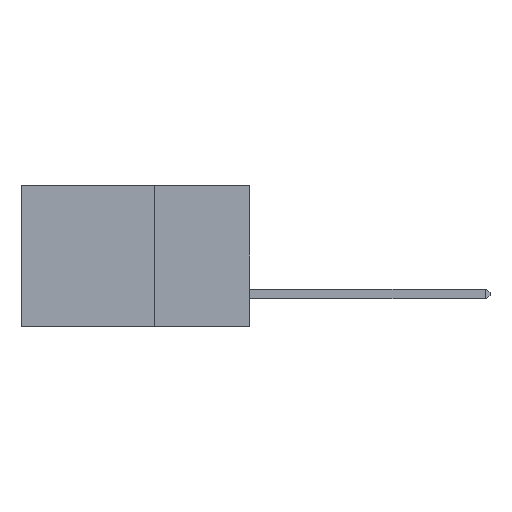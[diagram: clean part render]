
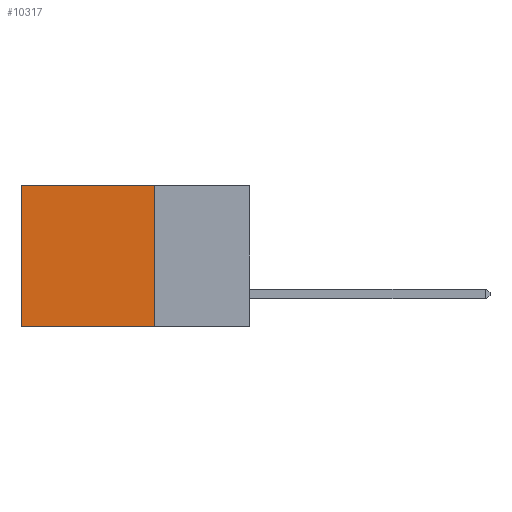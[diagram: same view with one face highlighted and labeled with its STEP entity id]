
A CAD part, left-side view. The second image highlights one B-rep face of the part: STEP entity #10317.
In plain terms, the highlighted planar face has unit normal (-1, 0, 0).
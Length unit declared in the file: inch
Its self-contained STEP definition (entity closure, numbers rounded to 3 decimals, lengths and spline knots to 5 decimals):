
#121 = PLANE ( 'NONE',  #26026 ) ;
#362 = VECTOR ( 'NONE', #3982, 39.37008 ) ;
#549 = DIRECTION ( 'NONE',  ( 0., 1., 0. ) ) ;
#774 = CARTESIAN_POINT ( 'NONE',  ( 0.2875, 0.25, 0. ) ) ;
#946 = EDGE_LOOP ( 'NONE', ( #1209, #22316, #26068, #19236 ) ) ;
#1209 = ORIENTED_EDGE ( 'NONE', *, *, #5590, .T. ) ;
#3982 = DIRECTION ( 'NONE',  ( 0., 0., -1. ) ) ;
#4179 = VERTEX_POINT ( 'NONE', #16842 ) ;
#4461 = DIRECTION ( 'NONE',  ( 0., 0., -1. ) ) ;
#5590 = EDGE_CURVE ( 'NONE', #4179, #8663, #16687, .T. ) ;
#5706 = LINE ( 'NONE', #15472, #21201 ) ;
#5840 = VERTEX_POINT ( 'NONE', #25063 ) ;
#7471 = CARTESIAN_POINT ( 'NONE',  ( 0.2875, 0.6, 0. ) ) ;
#8360 = CARTESIAN_POINT ( 'NONE',  ( 0.2875, 0.25, 0. ) ) ;
#8663 = VERTEX_POINT ( 'NONE', #9883 ) ;
#9883 = CARTESIAN_POINT ( 'NONE',  ( 0.2875, 0.6, -0.37 ) ) ;
#10317 = ADVANCED_FACE ( 'NONE', ( #17833 ), #121, .F. ) ;
#10631 = DIRECTION ( 'NONE',  ( 0., 1., 0. ) ) ;
#11395 = VECTOR ( 'NONE', #10631, 39.37008 ) ;
#13934 = VERTEX_POINT ( 'NONE', #774 ) ;
#14604 = CARTESIAN_POINT ( 'NONE',  ( 0.2875, 0.25, 0. ) ) ;
#15472 = CARTESIAN_POINT ( 'NONE',  ( 0.2875, 0.25, -0.37 ) ) ;
#16010 = EDGE_CURVE ( 'NONE', #13934, #5840, #17358, .T. ) ;
#16028 = VECTOR ( 'NONE', #20110, 39.37008 ) ;
#16687 = LINE ( 'NONE', #7471, #16028 ) ;
#16730 = EDGE_CURVE ( 'NONE', #5840, #8663, #5706, .T. ) ;
#16842 = CARTESIAN_POINT ( 'NONE',  ( 0.2875, 0.6, 0. ) ) ;
#16971 = LINE ( 'NONE', #8360, #11395 ) ;
#17167 = DIRECTION ( 'NONE',  ( 1., 0., 0. ) ) ;
#17358 = LINE ( 'NONE', #14604, #362 ) ;
#17833 = FACE_OUTER_BOUND ( 'NONE', #946, .T. ) ;
#19236 = ORIENTED_EDGE ( 'NONE', *, *, #25788, .T. ) ;
#20110 = DIRECTION ( 'NONE',  ( 0., 0., -1. ) ) ;
#21201 = VECTOR ( 'NONE', #549, 39.37008 ) ;
#22316 = ORIENTED_EDGE ( 'NONE', *, *, #16730, .F. ) ;
#25063 = CARTESIAN_POINT ( 'NONE',  ( 0.2875, 0.25, -0.37 ) ) ;
#25383 = CARTESIAN_POINT ( 'NONE',  ( 0.2875, 0.25, 0. ) ) ;
#25788 = EDGE_CURVE ( 'NONE', #13934, #4179, #16971, .T. ) ;
#26026 = AXIS2_PLACEMENT_3D ( 'NONE', #25383, #17167, #4461 ) ;
#26068 = ORIENTED_EDGE ( 'NONE', *, *, #16010, .F. ) ;
